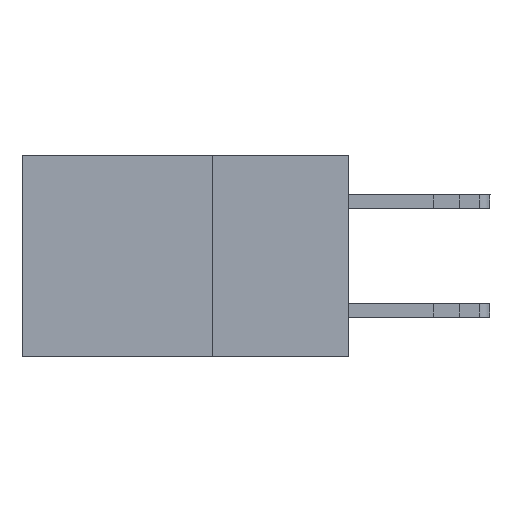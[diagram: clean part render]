
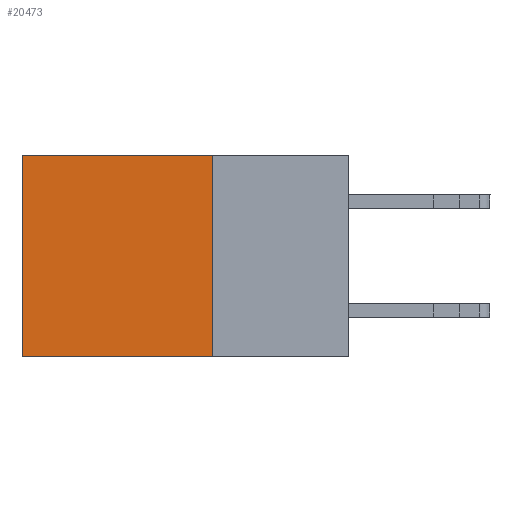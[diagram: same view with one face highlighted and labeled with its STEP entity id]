
A CAD part, left-side view. The second image highlights one B-rep face of the part: STEP entity #20473.
In plain terms, the highlighted planar face has unit normal (-1, 0, 0).
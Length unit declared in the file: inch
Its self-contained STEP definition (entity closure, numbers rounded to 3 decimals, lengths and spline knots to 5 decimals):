
#144 = VECTOR ( 'NONE', #1690, 39.37008 ) ;
#217 = PLANE ( 'NONE',  #22181 ) ;
#266 = LINE ( 'NONE', #18927, #26525 ) ;
#1042 = EDGE_CURVE ( 'NONE', #9079, #4481, #9168, .T. ) ;
#1690 = DIRECTION ( 'NONE',  ( 0., 0., -1. ) ) ;
#4481 = VERTEX_POINT ( 'NONE', #9171 ) ;
#4496 = ORIENTED_EDGE ( 'NONE', *, *, #17210, .F. ) ;
#5544 = CARTESIAN_POINT ( 'NONE',  ( 0.298, 0.6, -0.37 ) ) ;
#5994 = CARTESIAN_POINT ( 'NONE',  ( 0.298, 0.25, 0. ) ) ;
#7078 = CARTESIAN_POINT ( 'NONE',  ( 0.298, 0.25, 0. ) ) ;
#7601 = ORIENTED_EDGE ( 'NONE', *, *, #16724, .F. ) ;
#8625 = DIRECTION ( 'NONE',  ( 0., 0., -1. ) ) ;
#9079 = VERTEX_POINT ( 'NONE', #20803 ) ;
#9168 = LINE ( 'NONE', #7078, #27068 ) ;
#9171 = CARTESIAN_POINT ( 'NONE',  ( 0.298, 0.6, 0. ) ) ;
#9487 = CARTESIAN_POINT ( 'NONE',  ( 0.298, 0.25, -0.37 ) ) ;
#12321 = CARTESIAN_POINT ( 'NONE',  ( 0.298, 0.25, 0. ) ) ;
#12613 = CARTESIAN_POINT ( 'NONE',  ( 0.298, 0.6, 0. ) ) ;
#14041 = ORIENTED_EDGE ( 'NONE', *, *, #20930, .T. ) ;
#15525 = DIRECTION ( 'NONE',  ( 0., 1., 0. ) ) ;
#15915 = EDGE_LOOP ( 'NONE', ( #14041, #4496, #7601, #21485 ) ) ;
#16059 = LINE ( 'NONE', #12321, #22485 ) ;
#16724 = EDGE_CURVE ( 'NONE', #9079, #23723, #16059, .T. ) ;
#17210 = EDGE_CURVE ( 'NONE', #23723, #26031, #266, .T. ) ;
#18787 = DIRECTION ( 'NONE',  ( 0., 1., 0. ) ) ;
#18927 = CARTESIAN_POINT ( 'NONE',  ( 0.298, 0.25, -0.37 ) ) ;
#20473 = ADVANCED_FACE ( 'NONE', ( #24993 ), #217, .F. ) ;
#20803 = CARTESIAN_POINT ( 'NONE',  ( 0.298, 0.25, 0. ) ) ;
#20930 = EDGE_CURVE ( 'NONE', #4481, #26031, #25094, .T. ) ;
#21485 = ORIENTED_EDGE ( 'NONE', *, *, #1042, .T. ) ;
#22181 = AXIS2_PLACEMENT_3D ( 'NONE', #5994, #23052, #8625 ) ;
#22485 = VECTOR ( 'NONE', #24518, 39.37008 ) ;
#23052 = DIRECTION ( 'NONE',  ( 1., 0., 0. ) ) ;
#23723 = VERTEX_POINT ( 'NONE', #9487 ) ;
#24518 = DIRECTION ( 'NONE',  ( 0., 0., -1. ) ) ;
#24993 = FACE_OUTER_BOUND ( 'NONE', #15915, .T. ) ;
#25094 = LINE ( 'NONE', #12613, #144 ) ;
#26031 = VERTEX_POINT ( 'NONE', #5544 ) ;
#26525 = VECTOR ( 'NONE', #18787, 39.37008 ) ;
#27068 = VECTOR ( 'NONE', #15525, 39.37008 ) ;
